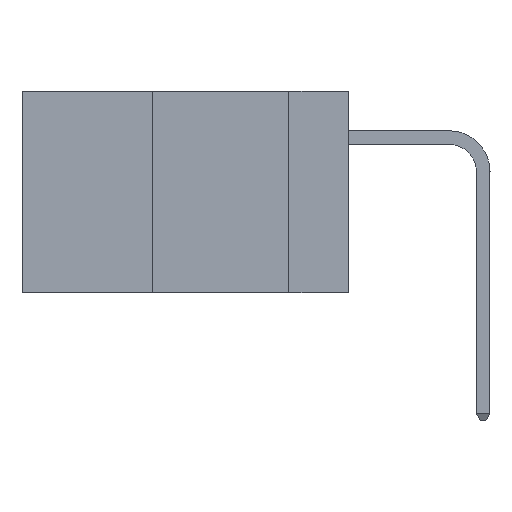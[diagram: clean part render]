
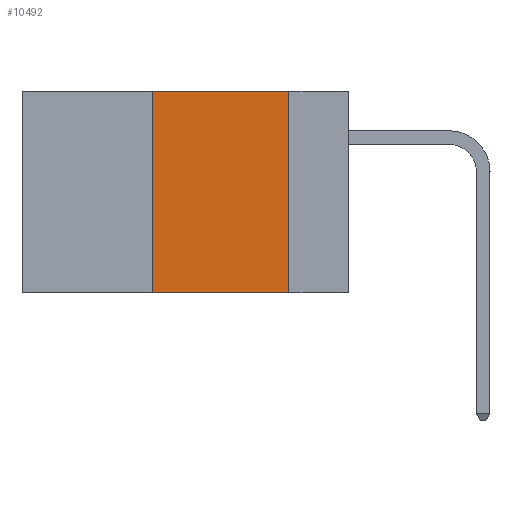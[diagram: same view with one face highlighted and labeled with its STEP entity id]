
A CAD part, left-side view. The second image highlights one B-rep face of the part: STEP entity #10492.
In plain terms, the highlighted planar face has unit normal (-1, 0, 0).
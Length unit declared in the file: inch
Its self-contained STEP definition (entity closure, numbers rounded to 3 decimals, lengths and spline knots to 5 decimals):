
#822 = CARTESIAN_POINT ( 'NONE',  ( 0., 0.6, 0. ) ) ;
#841 = LINE ( 'NONE', #11467, #9098 ) ;
#2446 = VECTOR ( 'NONE', #18972, 39.37008 ) ;
#2781 = ORIENTED_EDGE ( 'NONE', *, *, #9435, .T. ) ;
#4246 = VERTEX_POINT ( 'NONE', #10925 ) ;
#4942 = FACE_OUTER_BOUND ( 'NONE', #5031, .T. ) ;
#5027 = EDGE_CURVE ( 'NONE', #4246, #7811, #11137, .T. ) ;
#5031 = EDGE_LOOP ( 'NONE', ( #17275, #14640, #18719, #2781 ) ) ;
#5644 = CARTESIAN_POINT ( 'NONE',  ( 0., 0.6, 0. ) ) ;
#6088 = EDGE_CURVE ( 'NONE', #13655, #16785, #15507, .T. ) ;
#7225 = LINE ( 'NONE', #5644, #15262 ) ;
#7455 = PLANE ( 'NONE',  #14522 ) ;
#7811 = VERTEX_POINT ( 'NONE', #9140 ) ;
#8274 = DIRECTION ( 'NONE',  ( 0., -1., 0. ) ) ;
#9074 = CARTESIAN_POINT ( 'NONE',  ( 0., 0.36, -0.37 ) ) ;
#9098 = VECTOR ( 'NONE', #8274, 39.37008 ) ;
#9121 = DIRECTION ( 'NONE',  ( 0., 0., -1. ) ) ;
#9140 = CARTESIAN_POINT ( 'NONE',  ( 0., 0.11, -0.37 ) ) ;
#9435 = EDGE_CURVE ( 'NONE', #13655, #7811, #841, .T. ) ;
#9447 = CARTESIAN_POINT ( 'NONE',  ( 0., 0.36, 0. ) ) ;
#10492 = ADVANCED_FACE ( 'NONE', ( #4942 ), #7455, .F. ) ;
#10925 = CARTESIAN_POINT ( 'NONE',  ( 0., 0.11, 0. ) ) ;
#11066 = DIRECTION ( 'NONE',  ( 0., 0., 1. ) ) ;
#11137 = LINE ( 'NONE', #15893, #2446 ) ;
#11328 = VECTOR ( 'NONE', #11066, 39.37008 ) ;
#11467 = CARTESIAN_POINT ( 'NONE',  ( 0., 0.6, -0.37 ) ) ;
#13655 = VERTEX_POINT ( 'NONE', #9074 ) ;
#13721 = DIRECTION ( 'NONE',  ( 0., -1., 0. ) ) ;
#14522 = AXIS2_PLACEMENT_3D ( 'NONE', #822, #18499, #9121 ) ;
#14640 = ORIENTED_EDGE ( 'NONE', *, *, #19351, .F. ) ;
#15262 = VECTOR ( 'NONE', #13721, 39.37008 ) ;
#15507 = LINE ( 'NONE', #9447, #11328 ) ;
#15893 = CARTESIAN_POINT ( 'NONE',  ( 0., 0.11, 0. ) ) ;
#16122 = CARTESIAN_POINT ( 'NONE',  ( 0., 0.36, 0. ) ) ;
#16785 = VERTEX_POINT ( 'NONE', #16122 ) ;
#17275 = ORIENTED_EDGE ( 'NONE', *, *, #5027, .F. ) ;
#18499 = DIRECTION ( 'NONE',  ( 1., 0., 0. ) ) ;
#18719 = ORIENTED_EDGE ( 'NONE', *, *, #6088, .F. ) ;
#18972 = DIRECTION ( 'NONE',  ( 0., 0., -1. ) ) ;
#19351 = EDGE_CURVE ( 'NONE', #16785, #4246, #7225, .T. ) ;
